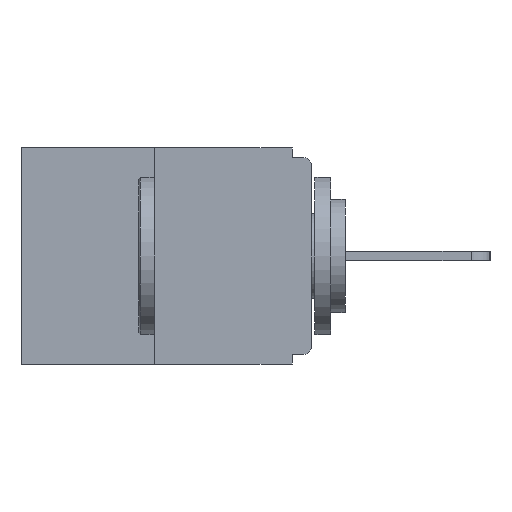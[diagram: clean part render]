
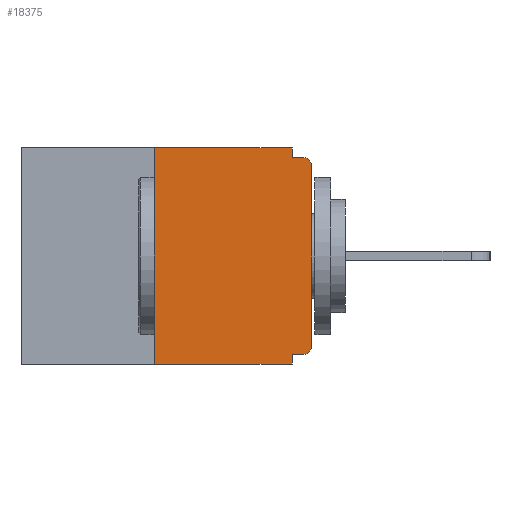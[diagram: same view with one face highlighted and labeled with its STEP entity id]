
A CAD part, left-side view. The second image highlights one B-rep face of the part: STEP entity #18375.
In plain terms, the highlighted planar face has unit normal (-1, 0, 0).
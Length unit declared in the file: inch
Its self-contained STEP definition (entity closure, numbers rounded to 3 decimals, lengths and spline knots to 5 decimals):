
#294 = VECTOR ( 'NONE', #16860, 39.37008 ) ;
#363 = ORIENTED_EDGE ( 'NONE', *, *, #26579, .F. ) ;
#1138 = VERTEX_POINT ( 'NONE', #8594 ) ;
#1329 = VERTEX_POINT ( 'NONE', #24505 ) ;
#1530 = EDGE_CURVE ( 'NONE', #9289, #24405, #6440, .T. ) ;
#1576 = CARTESIAN_POINT ( 'NONE',  ( 0., 0.031, -0.015 ) ) ;
#2000 = CARTESIAN_POINT ( 'NONE',  ( 0., 0.46, 0. ) ) ;
#2190 = ORIENTED_EDGE ( 'NONE', *, *, #1530, .F. ) ;
#2623 = VERTEX_POINT ( 'NONE', #12077 ) ;
#2765 = DIRECTION ( 'NONE',  ( 0., 0., -1. ) ) ;
#3044 = CARTESIAN_POINT ( 'NONE',  ( 0., 0.015, -0.03 ) ) ;
#3250 = DIRECTION ( 'NONE',  ( 0., 0., -1. ) ) ;
#4276 = AXIS2_PLACEMENT_3D ( 'NONE', #3044, #17682, #2765 ) ;
#4696 = AXIS2_PLACEMENT_3D ( 'NONE', #14713, #22811, #16936 ) ;
#5410 = EDGE_CURVE ( 'NONE', #18389, #19348, #20178, .T. ) ;
#5745 = CARTESIAN_POINT ( 'NONE',  ( 0., 0.46, 0. ) ) ;
#6126 = VECTOR ( 'NONE', #13774, 39.37008 ) ;
#6222 = ORIENTED_EDGE ( 'NONE', *, *, #5410, .F. ) ;
#6440 = LINE ( 'NONE', #17438, #21976 ) ;
#7704 = PLANE ( 'NONE',  #13498 ) ;
#7835 = CIRCLE ( 'NONE', #4696, 0.015 ) ;
#8121 = EDGE_CURVE ( 'NONE', #16866, #18389, #19355, .T. ) ;
#8212 = VECTOR ( 'NONE', #19416, 39.37008 ) ;
#8296 = EDGE_CURVE ( 'NONE', #10051, #19348, #10128, .T. ) ;
#8594 = CARTESIAN_POINT ( 'NONE',  ( 0., 0.015, -0.328 ) ) ;
#8673 = DIRECTION ( 'NONE',  ( 0., -1., 0. ) ) ;
#9289 = VERTEX_POINT ( 'NONE', #13039 ) ;
#9709 = ORIENTED_EDGE ( 'NONE', *, *, #21741, .T. ) ;
#10051 = VERTEX_POINT ( 'NONE', #19527 ) ;
#10111 = ORIENTED_EDGE ( 'NONE', *, *, #15469, .F. ) ;
#10128 = CIRCLE ( 'NONE', #4276, 0.015 ) ;
#10492 = LINE ( 'NONE', #2000, #22262 ) ;
#10903 = VECTOR ( 'NONE', #26781, 39.37008 ) ;
#11132 = EDGE_LOOP ( 'NONE', ( #363, #10111, #27004, #2190, #25991, #12248, #9709, #20512, #6222, #25185 ) ) ;
#12077 = CARTESIAN_POINT ( 'NONE',  ( 0., 0., -0.313 ) ) ;
#12131 = LINE ( 'NONE', #23010, #10903 ) ;
#12248 = ORIENTED_EDGE ( 'NONE', *, *, #22195, .T. ) ;
#13039 = CARTESIAN_POINT ( 'NONE',  ( 0., 0.031, -0.328 ) ) ;
#13159 = CARTESIAN_POINT ( 'NONE',  ( 0., 0.25, 0. ) ) ;
#13282 = CARTESIAN_POINT ( 'NONE',  ( 0., 0.46, -0.343 ) ) ;
#13498 = AXIS2_PLACEMENT_3D ( 'NONE', #5745, #13844, #3250 ) ;
#13774 = DIRECTION ( 'NONE',  ( 0., -1., 0. ) ) ;
#13788 = EDGE_CURVE ( 'NONE', #1329, #24405, #24140, .T. ) ;
#13844 = DIRECTION ( 'NONE',  ( 1., 0., 0. ) ) ;
#14301 = CARTESIAN_POINT ( 'NONE',  ( 0., 0., -0.328 ) ) ;
#14601 = VECTOR ( 'NONE', #26834, 39.37008 ) ;
#14713 = CARTESIAN_POINT ( 'NONE',  ( 0., 0.015, -0.313 ) ) ;
#14820 = VERTEX_POINT ( 'NONE', #21304 ) ;
#15469 = EDGE_CURVE ( 'NONE', #1329, #14820, #23747, .T. ) ;
#16860 = DIRECTION ( 'NONE',  ( 0., 0., -1. ) ) ;
#16866 = VERTEX_POINT ( 'NONE', #23194 ) ;
#16936 = DIRECTION ( 'NONE',  ( 0., 0., -1. ) ) ;
#17397 = CARTESIAN_POINT ( 'NONE',  ( 0., 0.031, 0. ) ) ;
#17438 = CARTESIAN_POINT ( 'NONE',  ( 0., 0.031, -0.343 ) ) ;
#17682 = DIRECTION ( 'NONE',  ( -1., 0., 0. ) ) ;
#18062 = LINE ( 'NONE', #14301, #14601 ) ;
#18375 = ADVANCED_FACE ( 'NONE', ( #26935 ), #7704, .F. ) ;
#18389 = VERTEX_POINT ( 'NONE', #1576 ) ;
#19348 = VERTEX_POINT ( 'NONE', #26432 ) ;
#19355 = LINE ( 'NONE', #17397, #294 ) ;
#19416 = DIRECTION ( 'NONE',  ( 0., -1., 0. ) ) ;
#19527 = CARTESIAN_POINT ( 'NONE',  ( 0., 0., -0.03 ) ) ;
#19864 = VECTOR ( 'NONE', #24880, 39.37008 ) ;
#20178 = LINE ( 'NONE', #24648, #6126 ) ;
#20512 = ORIENTED_EDGE ( 'NONE', *, *, #8296, .T. ) ;
#21304 = CARTESIAN_POINT ( 'NONE',  ( 0., 0.25, 0. ) ) ;
#21741 = EDGE_CURVE ( 'NONE', #2623, #10051, #12131, .T. ) ;
#21976 = VECTOR ( 'NONE', #25951, 39.37008 ) ;
#22195 = EDGE_CURVE ( 'NONE', #1138, #2623, #7835, .T. ) ;
#22262 = VECTOR ( 'NONE', #8673, 39.37008 ) ;
#22811 = DIRECTION ( 'NONE',  ( -1., 0., 0. ) ) ;
#23010 = CARTESIAN_POINT ( 'NONE',  ( 0., 0., 0. ) ) ;
#23194 = CARTESIAN_POINT ( 'NONE',  ( 0., 0.031, 0. ) ) ;
#23747 = LINE ( 'NONE', #13159, #19864 ) ;
#24140 = LINE ( 'NONE', #13282, #8212 ) ;
#24405 = VERTEX_POINT ( 'NONE', #25875 ) ;
#24498 = EDGE_CURVE ( 'NONE', #1138, #9289, #18062, .T. ) ;
#24505 = CARTESIAN_POINT ( 'NONE',  ( 0., 0.25, -0.343 ) ) ;
#24648 = CARTESIAN_POINT ( 'NONE',  ( 0., 0., -0.015 ) ) ;
#24880 = DIRECTION ( 'NONE',  ( 0., 0., 1. ) ) ;
#25185 = ORIENTED_EDGE ( 'NONE', *, *, #8121, .F. ) ;
#25875 = CARTESIAN_POINT ( 'NONE',  ( 0., 0.031, -0.343 ) ) ;
#25951 = DIRECTION ( 'NONE',  ( 0., 0., -1. ) ) ;
#25991 = ORIENTED_EDGE ( 'NONE', *, *, #24498, .F. ) ;
#26432 = CARTESIAN_POINT ( 'NONE',  ( 0., 0.015, -0.015 ) ) ;
#26579 = EDGE_CURVE ( 'NONE', #14820, #16866, #10492, .T. ) ;
#26781 = DIRECTION ( 'NONE',  ( 0., 0., 1. ) ) ;
#26834 = DIRECTION ( 'NONE',  ( 0., 1., 0. ) ) ;
#26935 = FACE_OUTER_BOUND ( 'NONE', #11132, .T. ) ;
#27004 = ORIENTED_EDGE ( 'NONE', *, *, #13788, .T. ) ;
